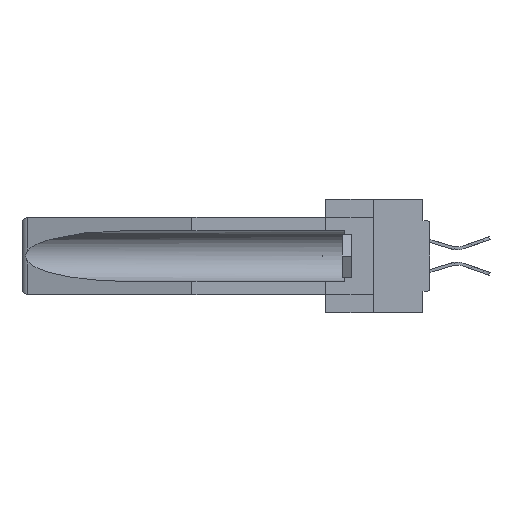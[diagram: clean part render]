
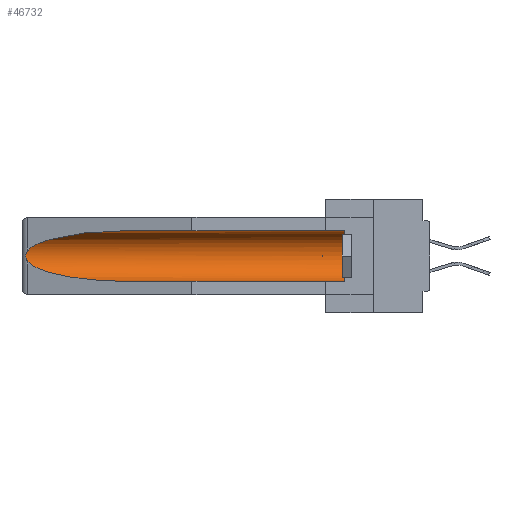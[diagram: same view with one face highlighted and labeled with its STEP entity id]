
A CAD part, left-side view. The second image highlights one B-rep face of the part: STEP entity #46732.
In plain terms, the highlighted cylindrical face has radius 2.857 mm (diameter 5.715 mm), a partial arc.
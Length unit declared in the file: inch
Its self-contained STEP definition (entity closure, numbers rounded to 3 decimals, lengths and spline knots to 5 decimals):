
#568 = CIRCLE ( 'NONE', #44431, 0.1125 ) ;
#804 = EDGE_CURVE ( 'NONE', #42016, #17140, #568, .T. ) ;
#1930 = DIRECTION ( 'NONE',  ( 0., 0., 1. ) ) ;
#3036 = CARTESIAN_POINT ( 'NONE',  ( 0.26537, 1.52718, -0.19328 ) ) ;
#3248 = CARTESIAN_POINT ( 'NONE',  ( 0.155, -0.30754, -0.284 ) ) ;
#3286 = EDGE_CURVE ( 'NONE', #31664, #23335, #32027, .T. ) ;
#3313 = CARTESIAN_POINT ( 'NONE',  ( 0.25451, 1.48313, -0.09465 ) ) ;
#3511 =( BOUNDED_CURVE ( )  B_SPLINE_CURVE ( 3, ( #27700, #38825, #42731, #5123 ),
 .UNSPECIFIED., .F., .T. ) 
 B_SPLINE_CURVE_WITH_KNOTS ( ( 4, 4 ),
 ( 0.1948, 1.5708 ),
 .UNSPECIFIED. ) 
 CURVE ( )  GEOMETRIC_REPRESENTATION_ITEM ( )  RATIONAL_B_SPLINE_CURVE ( ( 1., 0.848, 0.848, 1. ) ) 
 REPRESENTATION_ITEM ( '' )  );
#4220 = DIRECTION ( 'NONE',  ( 0., -1., 0. ) ) ;
#4971 = CARTESIAN_POINT ( 'NONE',  ( 0.155, 0.126, -0.059 ) ) ;
#5123 = CARTESIAN_POINT ( 'NONE',  ( 0.155, 1.07973, -0.284 ) ) ;
#7425 = ORIENTED_EDGE ( 'NONE', *, *, #33912, .T. ) ;
#7792 = CARTESIAN_POINT ( 'NONE',  ( 0.155, -0.30754, -0.1715 ) ) ;
#8495 = VECTOR ( 'NONE', #21585, 39.37008 ) ;
#10428 = CARTESIAN_POINT ( 'NONE',  ( 0.26597, 1.52961, -0.15275 ) ) ;
#10582 = CARTESIAN_POINT ( 'NONE',  ( 0.26655, 1.53094, -0.18657 ) ) ;
#12218 =( BOUNDED_CURVE ( )  B_SPLINE_CURVE ( 3, ( #33586, #45016, #3313, #29481 ),
 .UNSPECIFIED., .F., .F. ) 
 B_SPLINE_CURVE_WITH_KNOTS ( ( 4, 4 ),
 ( 4.71239, 6.08839 ),
 .UNSPECIFIED. ) 
 CURVE ( )  GEOMETRIC_REPRESENTATION_ITEM ( )  RATIONAL_B_SPLINE_CURVE ( ( 1., 0.848, 0.848, 1. ) ) 
 REPRESENTATION_ITEM ( '' )  );
#13323 = FACE_OUTER_BOUND ( 'NONE', #21811, .T. ) ;
#13644 = ORIENTED_EDGE ( 'NONE', *, *, #35796, .T. ) ;
#14150 = CARTESIAN_POINT ( 'NONE',  ( 0.2673, 1.5327, -0.16383 ) ) ;
#14786 = CARTESIAN_POINT ( 'NONE',  ( 0.26537, 1.52718, -0.14972 ) ) ;
#17140 = VERTEX_POINT ( 'NONE', #4971 ) ;
#17952 = CARTESIAN_POINT ( 'NONE',  ( 0.2673, 1.53269, -0.17917 ) ) ;
#19728 = ORIENTED_EDGE ( 'NONE', *, *, #38586, .T. ) ;
#21585 = DIRECTION ( 'NONE',  ( 0., 1., 0. ) ) ;
#21671 = CARTESIAN_POINT ( 'NONE',  ( 0.26597, 1.5296, -0.19026 ) ) ;
#21714 = EDGE_CURVE ( 'NONE', #42016, #34630, #34276, .T. ) ;
#21811 = EDGE_LOOP ( 'NONE', ( #7425, #26469, #13644, #47721, #35267, #19728 ) ) ;
#21842 = CARTESIAN_POINT ( 'NONE',  ( 0.2675, 1.53308, -0.16763 ) ) ;
#23335 = VERTEX_POINT ( 'NONE', #37754 ) ;
#23727 = CARTESIAN_POINT ( 'NONE',  ( 0.155, 1.07973, -0.284 ) ) ;
#24475 = CYLINDRICAL_SURFACE ( 'NONE', #26879, 0.1125 ) ;
#25752 = VECTOR ( 'NONE', #35212, 39.37008 ) ;
#26469 = ORIENTED_EDGE ( 'NONE', *, *, #3286, .T. ) ;
#26637 = CARTESIAN_POINT ( 'NONE',  ( 0.155, 0.126, -0.1715 ) ) ;
#26879 = AXIS2_PLACEMENT_3D ( 'NONE', #7792, #34122, #34297 ) ;
#27700 = CARTESIAN_POINT ( 'NONE',  ( 0.26537, 1.52718, -0.19328 ) ) ;
#28172 = CARTESIAN_POINT ( 'NONE',  ( 0.155, -0.30754, -0.059 ) ) ;
#29481 = CARTESIAN_POINT ( 'NONE',  ( 0.26537, 1.52718, -0.14972 ) ) ;
#31664 = VERTEX_POINT ( 'NONE', #32317 ) ;
#32027 = B_SPLINE_CURVE_WITH_KNOTS ( 'NONE', 3,
 ( #14786, #10428, #36573, #14150, #21842, #32995, #17952, #10582, #21671, #3036 ),
 .UNSPECIFIED., .F., .F.,
 ( 4, 2, 2, 2, 4 ),
 ( 0., 0.00029, 0.00058, 0.00087, 0.00117 ),
 .UNSPECIFIED. ) ;
#32317 = CARTESIAN_POINT ( 'NONE',  ( 0.26537, 1.52718, -0.14972 ) ) ;
#32995 = CARTESIAN_POINT ( 'NONE',  ( 0.2675, 1.53308, -0.17534 ) ) ;
#33586 = CARTESIAN_POINT ( 'NONE',  ( 0.155, 1.07973, -0.059 ) ) ;
#33912 = EDGE_CURVE ( 'NONE', #46696, #31664, #12218, .T. ) ;
#34122 = DIRECTION ( 'NONE',  ( 0., 1., 0. ) ) ;
#34276 = LINE ( 'NONE', #3248, #8495 ) ;
#34297 = DIRECTION ( 'NONE',  ( 0., 0., 1. ) ) ;
#34630 = VERTEX_POINT ( 'NONE', #23727 ) ;
#35212 = DIRECTION ( 'NONE',  ( 0., 1., 0. ) ) ;
#35267 = ORIENTED_EDGE ( 'NONE', *, *, #804, .T. ) ;
#35725 = LINE ( 'NONE', #28172, #25752 ) ;
#35796 = EDGE_CURVE ( 'NONE', #23335, #34630, #3511, .T. ) ;
#36573 = CARTESIAN_POINT ( 'NONE',  ( 0.26654, 1.53092, -0.15636 ) ) ;
#37754 = CARTESIAN_POINT ( 'NONE',  ( 0.26537, 1.52718, -0.19328 ) ) ;
#38586 = EDGE_CURVE ( 'NONE', #17140, #46696, #35725, .T. ) ;
#38825 = CARTESIAN_POINT ( 'NONE',  ( 0.25451, 1.48313, -0.24835 ) ) ;
#39204 = CARTESIAN_POINT ( 'NONE',  ( 0.155, 0.126, -0.284 ) ) ;
#42016 = VERTEX_POINT ( 'NONE', #39204 ) ;
#42731 = CARTESIAN_POINT ( 'NONE',  ( 0.21114, 1.30732, -0.284 ) ) ;
#44431 = AXIS2_PLACEMENT_3D ( 'NONE', #26637, #4220, #1930 ) ;
#44927 = CARTESIAN_POINT ( 'NONE',  ( 0.155, 1.07973, -0.059 ) ) ;
#45016 = CARTESIAN_POINT ( 'NONE',  ( 0.21114, 1.30732, -0.059 ) ) ;
#46696 = VERTEX_POINT ( 'NONE', #44927 ) ;
#46732 = ADVANCED_FACE ( 'NONE', ( #13323 ), #24475, .F. ) ;
#47721 = ORIENTED_EDGE ( 'NONE', *, *, #21714, .F. ) ;
